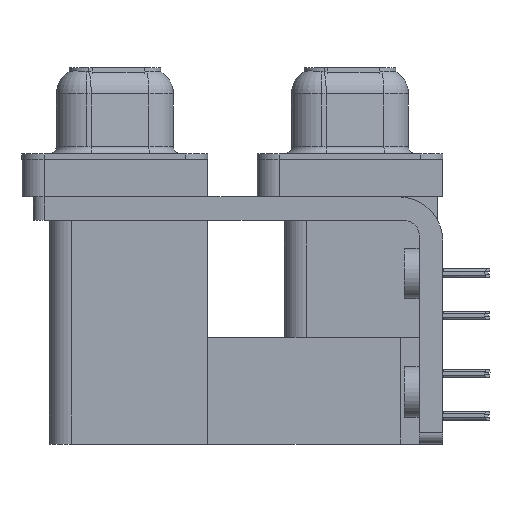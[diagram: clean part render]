
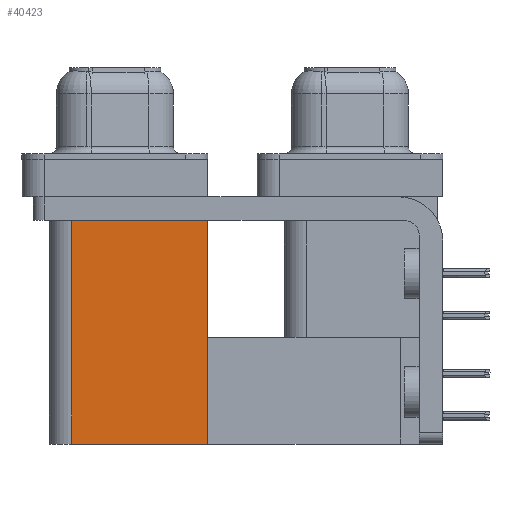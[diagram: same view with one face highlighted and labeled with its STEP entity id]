
A CAD part, left-side view. The second image highlights one B-rep face of the part: STEP entity #40423.
In plain terms, the highlighted planar face has unit normal (-1, 0, 0).
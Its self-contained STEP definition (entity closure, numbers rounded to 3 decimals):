
#677 = EDGE_CURVE ( 'NONE', #31908, #26498, #2100, .T. ) ;
#763 = DIRECTION ( 'NONE',  ( 0., 0., -1. ) ) ;
#2100 = LINE ( 'NONE', #18714, #40259 ) ;
#2577 = CARTESIAN_POINT ( 'NONE',  ( 3.765, 9.6, -19.2 ) ) ;
#8061 = FACE_OUTER_BOUND ( 'NONE', #12283, .T. ) ;
#8333 = CARTESIAN_POINT ( 'NONE',  ( 3.765, 9.6, -2.5 ) ) ;
#8840 = CARTESIAN_POINT ( 'NONE',  ( 3.765, 9.6, -19.2 ) ) ;
#12283 = EDGE_LOOP ( 'NONE', ( #48272, #14932, #47136, #33472 ) ) ;
#12431 = LINE ( 'NONE', #51318, #39256 ) ;
#14932 = ORIENTED_EDGE ( 'NONE', *, *, #45860, .F. ) ;
#15831 = VECTOR ( 'NONE', #17449, 1000. ) ;
#17449 = DIRECTION ( 'NONE',  ( 0., 1., 0. ) ) ;
#18714 = CARTESIAN_POINT ( 'NONE',  ( 3.765, 9.6, -19.2 ) ) ;
#20791 = PLANE ( 'NONE',  #32342 ) ;
#21596 = LINE ( 'NONE', #37680, #15831 ) ;
#26015 = DIRECTION ( 'NONE',  ( 0., 1., 0. ) ) ;
#26485 = VERTEX_POINT ( 'NONE', #8333 ) ;
#26498 = VERTEX_POINT ( 'NONE', #32212 ) ;
#27644 = CARTESIAN_POINT ( 'NONE',  ( 3.765, 18.8, -2.5 ) ) ;
#30032 = VECTOR ( 'NONE', #31007, 1000. ) ;
#31007 = DIRECTION ( 'NONE',  ( 0., 0., 1. ) ) ;
#31908 = VERTEX_POINT ( 'NONE', #2577 ) ;
#32212 = CARTESIAN_POINT ( 'NONE',  ( 3.765, 18.8, -19.2 ) ) ;
#32342 = AXIS2_PLACEMENT_3D ( 'NONE', #8840, #35840, #763 ) ;
#33472 = ORIENTED_EDGE ( 'NONE', *, *, #47750, .T. ) ;
#34639 = LINE ( 'NONE', #46327, #30032 ) ;
#35840 = DIRECTION ( 'NONE',  ( 1., 0., 0. ) ) ;
#37029 = VERTEX_POINT ( 'NONE', #27644 ) ;
#37680 = CARTESIAN_POINT ( 'NONE',  ( 3.765, 9.6, -2.5 ) ) ;
#39256 = VECTOR ( 'NONE', #39415, 1000. ) ;
#39415 = DIRECTION ( 'NONE',  ( 0., 0., 1. ) ) ;
#40259 = VECTOR ( 'NONE', #26015, 1000. ) ;
#40423 = ADVANCED_FACE ( 'NONE', ( #8061 ), #20791, .F. ) ;
#41165 = EDGE_CURVE ( 'NONE', #26485, #37029, #21596, .T. ) ;
#45860 = EDGE_CURVE ( 'NONE', #26498, #37029, #34639, .T. ) ;
#46327 = CARTESIAN_POINT ( 'NONE',  ( 3.765, 18.8, -19.2 ) ) ;
#47136 = ORIENTED_EDGE ( 'NONE', *, *, #677, .F. ) ;
#47750 = EDGE_CURVE ( 'NONE', #31908, #26485, #12431, .T. ) ;
#48272 = ORIENTED_EDGE ( 'NONE', *, *, #41165, .T. ) ;
#51318 = CARTESIAN_POINT ( 'NONE',  ( 3.765, 9.6, -19.2 ) ) ;
